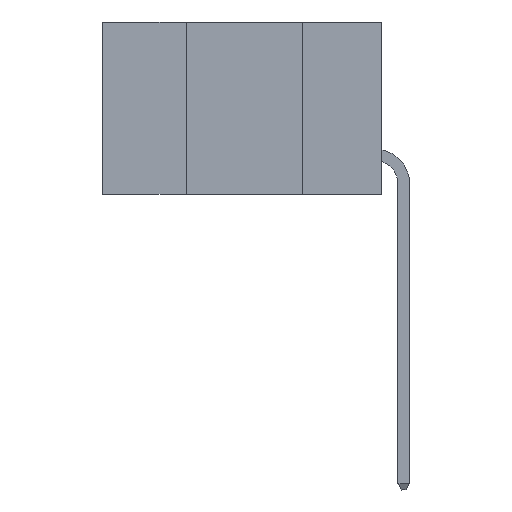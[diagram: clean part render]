
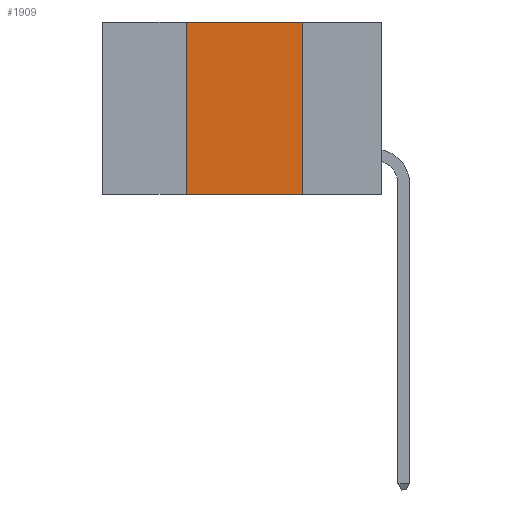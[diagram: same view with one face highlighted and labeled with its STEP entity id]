
A CAD part, left-side view. The second image highlights one B-rep face of the part: STEP entity #1909.
In plain terms, the highlighted planar face has unit normal (-1, 0, 0).
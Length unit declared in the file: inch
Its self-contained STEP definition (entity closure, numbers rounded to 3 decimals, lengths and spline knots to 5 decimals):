
#803 = EDGE_CURVE ( 'NONE', #7102, #4023, #14667, .T. ) ;
#1000 = FACE_OUTER_BOUND ( 'NONE', #10879, .T. ) ;
#1466 = VECTOR ( 'NONE', #7850, 39.37008 ) ;
#1909 = ADVANCED_FACE ( 'NONE', ( #1000 ), #3238, .F. ) ;
#2142 = EDGE_CURVE ( 'NONE', #5337, #7822, #14785, .T. ) ;
#2174 = CARTESIAN_POINT ( 'NONE',  ( 0., 0.42, 0. ) ) ;
#2344 = CARTESIAN_POINT ( 'NONE',  ( 0., 0.17, 0. ) ) ;
#3238 = PLANE ( 'NONE',  #8714 ) ;
#3337 = CARTESIAN_POINT ( 'NONE',  ( 0., 0.6, 0. ) ) ;
#3439 = VECTOR ( 'NONE', #13694, 39.37008 ) ;
#3561 = CARTESIAN_POINT ( 'NONE',  ( 0., 0.6, 0. ) ) ;
#4023 = VERTEX_POINT ( 'NONE', #2344 ) ;
#4229 = ORIENTED_EDGE ( 'NONE', *, *, #12598, .F. ) ;
#4546 = DIRECTION ( 'NONE',  ( 0., 0., -1. ) ) ;
#4726 = LINE ( 'NONE', #6713, #1466 ) ;
#5337 = VERTEX_POINT ( 'NONE', #5812 ) ;
#5812 = CARTESIAN_POINT ( 'NONE',  ( 0., 0.42, -0.37 ) ) ;
#6351 = CARTESIAN_POINT ( 'NONE',  ( 0., 0.17, -0.37 ) ) ;
#6539 = LINE ( 'NONE', #2174, #3439 ) ;
#6637 = EDGE_CURVE ( 'NONE', #5337, #7102, #6539, .T. ) ;
#6713 = CARTESIAN_POINT ( 'NONE',  ( 0., 0.17, 0. ) ) ;
#6841 = CARTESIAN_POINT ( 'NONE',  ( 0., 0.42, 0. ) ) ;
#7102 = VERTEX_POINT ( 'NONE', #6841 ) ;
#7657 = ORIENTED_EDGE ( 'NONE', *, *, #803, .F. ) ;
#7822 = VERTEX_POINT ( 'NONE', #6351 ) ;
#7850 = DIRECTION ( 'NONE',  ( 0., 0., -1. ) ) ;
#8011 = ORIENTED_EDGE ( 'NONE', *, *, #2142, .T. ) ;
#8059 = DIRECTION ( 'NONE',  ( 0., -1., 0. ) ) ;
#8714 = AXIS2_PLACEMENT_3D ( 'NONE', #3337, #11371, #4546 ) ;
#10879 = EDGE_LOOP ( 'NONE', ( #4229, #7657, #13640, #8011 ) ) ;
#11371 = DIRECTION ( 'NONE',  ( 1., 0., 0. ) ) ;
#11675 = VECTOR ( 'NONE', #8059, 39.37008 ) ;
#11746 = CARTESIAN_POINT ( 'NONE',  ( 0., 0.6, -0.37 ) ) ;
#11798 = VECTOR ( 'NONE', #12865, 39.37008 ) ;
#12598 = EDGE_CURVE ( 'NONE', #4023, #7822, #4726, .T. ) ;
#12865 = DIRECTION ( 'NONE',  ( 0., -1., 0. ) ) ;
#13640 = ORIENTED_EDGE ( 'NONE', *, *, #6637, .F. ) ;
#13694 = DIRECTION ( 'NONE',  ( 0., 0., 1. ) ) ;
#14667 = LINE ( 'NONE', #3561, #11675 ) ;
#14785 = LINE ( 'NONE', #11746, #11798 ) ;
